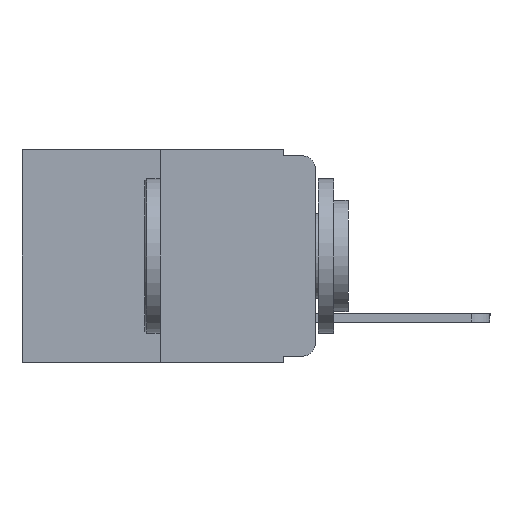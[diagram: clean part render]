
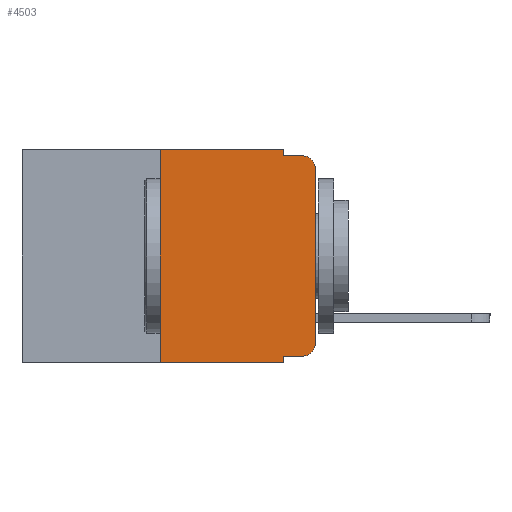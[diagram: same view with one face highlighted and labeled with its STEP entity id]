
A CAD part, left-side view. The second image highlights one B-rep face of the part: STEP entity #4503.
In plain terms, the highlighted planar face has unit normal (-1, 0, 0).
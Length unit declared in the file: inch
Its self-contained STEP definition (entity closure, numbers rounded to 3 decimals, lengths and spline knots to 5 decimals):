
#318 = DIRECTION ( 'NONE',  ( 0., 0., -1. ) ) ;
#592 = CARTESIAN_POINT ( 'NONE',  ( 0., 0.051, -0.333 ) ) ;
#660 = VERTEX_POINT ( 'NONE', #10713 ) ;
#951 = VERTEX_POINT ( 'NONE', #5433 ) ;
#1507 = VERTEX_POINT ( 'NONE', #12053 ) ;
#1725 = DIRECTION ( 'NONE',  ( 0., -1., 0. ) ) ;
#2213 = CARTESIAN_POINT ( 'NONE',  ( 0., 0., -0.03 ) ) ;
#2356 = VECTOR ( 'NONE', #11483, 39.37008 ) ;
#2531 = VERTEX_POINT ( 'NONE', #5103 ) ;
#2720 = LINE ( 'NONE', #5361, #5843 ) ;
#2911 = CARTESIAN_POINT ( 'NONE',  ( 0., 0., 0. ) ) ;
#2912 = ORIENTED_EDGE ( 'NONE', *, *, #9762, .F. ) ;
#3019 = CARTESIAN_POINT ( 'NONE',  ( 0., 0.051, -0.333 ) ) ;
#3095 = LINE ( 'NONE', #2911, #8529 ) ;
#3254 = ORIENTED_EDGE ( 'NONE', *, *, #9728, .T. ) ;
#3328 = ORIENTED_EDGE ( 'NONE', *, *, #9785, .T. ) ;
#3410 = CARTESIAN_POINT ( 'NONE',  ( 0., 0.051, -0.343 ) ) ;
#3852 = VERTEX_POINT ( 'NONE', #2213 ) ;
#4090 = DIRECTION ( 'NONE',  ( 0., 0., 1. ) ) ;
#4210 = CARTESIAN_POINT ( 'NONE',  ( 0., 0.25, 0. ) ) ;
#4263 = DIRECTION ( 'NONE',  ( -1., 0., 0. ) ) ;
#4503 = ADVANCED_FACE ( 'NONE', ( #13641 ), #12278, .F. ) ;
#4676 = VERTEX_POINT ( 'NONE', #6115 ) ;
#5103 = CARTESIAN_POINT ( 'NONE',  ( 0., 0., -0.313 ) ) ;
#5133 = VECTOR ( 'NONE', #12515, 39.37008 ) ;
#5316 = DIRECTION ( 'NONE',  ( 0., 0., -1. ) ) ;
#5329 = VERTEX_POINT ( 'NONE', #592 ) ;
#5361 = CARTESIAN_POINT ( 'NONE',  ( 0., 0.051, 0. ) ) ;
#5433 = CARTESIAN_POINT ( 'NONE',  ( 0., 0.02, -0.333 ) ) ;
#5514 = LINE ( 'NONE', #3019, #12952 ) ;
#5843 = VECTOR ( 'NONE', #5316, 39.37008 ) ;
#5885 = AXIS2_PLACEMENT_3D ( 'NONE', #13416, #7376, #318 ) ;
#6002 = VECTOR ( 'NONE', #11088, 39.37008 ) ;
#6115 = CARTESIAN_POINT ( 'NONE',  ( 0., 0.02, -0.01 ) ) ;
#6370 = CARTESIAN_POINT ( 'NONE',  ( 0., 0.051, -0.01 ) ) ;
#6825 = CARTESIAN_POINT ( 'NONE',  ( 0., 0.25, 0. ) ) ;
#7376 = DIRECTION ( 'NONE',  ( -1., 0., 0. ) ) ;
#7573 = CIRCLE ( 'NONE', #8585, 0.02 ) ;
#8529 = VECTOR ( 'NONE', #4090, 39.37008 ) ;
#8585 = AXIS2_PLACEMENT_3D ( 'NONE', #10574, #4263, #11537 ) ;
#8680 = LINE ( 'NONE', #10827, #13681 ) ;
#8853 = LINE ( 'NONE', #13451, #5133 ) ;
#9004 = EDGE_CURVE ( 'NONE', #12741, #660, #9028, .T. ) ;
#9010 = EDGE_LOOP ( 'NONE', ( #3254, #10460, #13394, #2912, #10008, #12823, #10034, #10524, #3328, #11598 ) ) ;
#9028 = LINE ( 'NONE', #9059, #6002 ) ;
#9059 = CARTESIAN_POINT ( 'NONE',  ( 0., 0.473, 0. ) ) ;
#9428 = EDGE_CURVE ( 'NONE', #1507, #13893, #8680, .T. ) ;
#9519 = DIRECTION ( 'NONE',  ( 0., -1., 0. ) ) ;
#9728 = EDGE_CURVE ( 'NONE', #2531, #3852, #3095, .T. ) ;
#9730 = EDGE_CURVE ( 'NONE', #3852, #4676, #11227, .T. ) ;
#9746 = EDGE_CURVE ( 'NONE', #13105, #4676, #13546, .T. ) ;
#9762 = EDGE_CURVE ( 'NONE', #660, #13105, #2720, .T. ) ;
#9764 = EDGE_CURVE ( 'NONE', #1507, #12741, #10631, .T. ) ;
#9765 = EDGE_CURVE ( 'NONE', #5329, #13893, #8853, .T. ) ;
#9785 = EDGE_CURVE ( 'NONE', #5329, #951, #5514, .T. ) ;
#9803 = EDGE_CURVE ( 'NONE', #951, #2531, #7573, .T. ) ;
#10008 = ORIENTED_EDGE ( 'NONE', *, *, #9004, .F. ) ;
#10034 = ORIENTED_EDGE ( 'NONE', *, *, #9428, .T. ) ;
#10460 = ORIENTED_EDGE ( 'NONE', *, *, #9730, .T. ) ;
#10524 = ORIENTED_EDGE ( 'NONE', *, *, #9765, .F. ) ;
#10574 = CARTESIAN_POINT ( 'NONE',  ( 0., 0.02, -0.313 ) ) ;
#10631 = LINE ( 'NONE', #4210, #2356 ) ;
#10713 = CARTESIAN_POINT ( 'NONE',  ( 0., 0.051, 0. ) ) ;
#10827 = CARTESIAN_POINT ( 'NONE',  ( 0., 0.473, -0.343 ) ) ;
#10922 = VECTOR ( 'NONE', #1725, 39.37008 ) ;
#11088 = DIRECTION ( 'NONE',  ( 0., -1., 0. ) ) ;
#11227 = CIRCLE ( 'NONE', #5885, 0.02 ) ;
#11483 = DIRECTION ( 'NONE',  ( 0., 0., 1. ) ) ;
#11537 = DIRECTION ( 'NONE',  ( 0., 0., -1. ) ) ;
#11598 = ORIENTED_EDGE ( 'NONE', *, *, #9803, .T. ) ;
#11769 = AXIS2_PLACEMENT_3D ( 'NONE', #13858, #13647, #13563 ) ;
#11815 = DIRECTION ( 'NONE',  ( 0., -1., 0. ) ) ;
#12053 = CARTESIAN_POINT ( 'NONE',  ( 0., 0.25, -0.343 ) ) ;
#12278 = PLANE ( 'NONE',  #11769 ) ;
#12297 = CARTESIAN_POINT ( 'NONE',  ( 0., 0.051, -0.01 ) ) ;
#12515 = DIRECTION ( 'NONE',  ( 0., 0., -1. ) ) ;
#12741 = VERTEX_POINT ( 'NONE', #6825 ) ;
#12823 = ORIENTED_EDGE ( 'NONE', *, *, #9764, .F. ) ;
#12952 = VECTOR ( 'NONE', #9519, 39.37008 ) ;
#13105 = VERTEX_POINT ( 'NONE', #12297 ) ;
#13394 = ORIENTED_EDGE ( 'NONE', *, *, #9746, .F. ) ;
#13416 = CARTESIAN_POINT ( 'NONE',  ( 0., 0.02, -0.03 ) ) ;
#13451 = CARTESIAN_POINT ( 'NONE',  ( 0., 0.051, 0. ) ) ;
#13546 = LINE ( 'NONE', #6370, #10922 ) ;
#13563 = DIRECTION ( 'NONE',  ( 0., 0., -1. ) ) ;
#13641 = FACE_OUTER_BOUND ( 'NONE', #9010, .T. ) ;
#13647 = DIRECTION ( 'NONE',  ( 1., 0., 0. ) ) ;
#13681 = VECTOR ( 'NONE', #11815, 39.37008 ) ;
#13858 = CARTESIAN_POINT ( 'NONE',  ( 0., 0.473, 0. ) ) ;
#13893 = VERTEX_POINT ( 'NONE', #3410 ) ;
